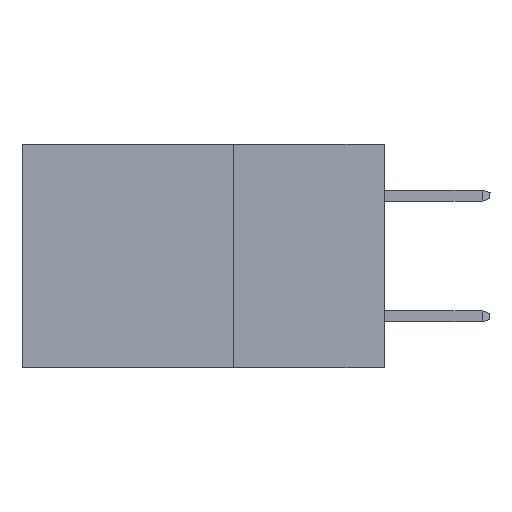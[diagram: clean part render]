
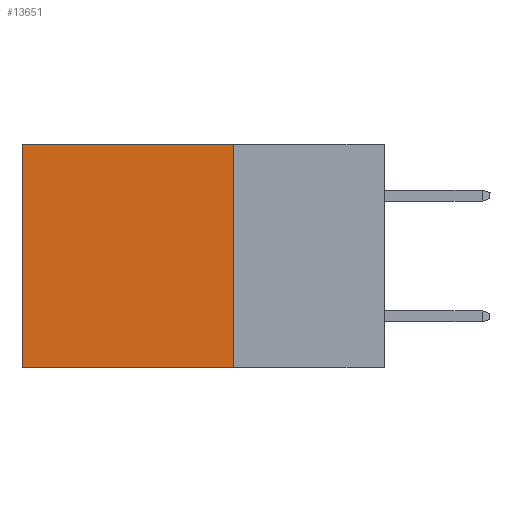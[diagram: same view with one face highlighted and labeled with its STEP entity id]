
A CAD part, left-side view. The second image highlights one B-rep face of the part: STEP entity #13651.
In plain terms, the highlighted planar face has unit normal (-1, 0, 0).
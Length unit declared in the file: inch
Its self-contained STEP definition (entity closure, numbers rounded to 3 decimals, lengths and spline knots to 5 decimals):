
#188 = VERTEX_POINT ( 'NONE', #18555 ) ;
#229 = VERTEX_POINT ( 'NONE', #8361 ) ;
#421 = LINE ( 'NONE', #22026, #21901 ) ;
#2353 = PLANE ( 'NONE',  #11314 ) ;
#4172 = DIRECTION ( 'NONE',  ( 0., 0., -1. ) ) ;
#4690 = CARTESIAN_POINT ( 'NONE',  ( 0.2615, 0.6, 0. ) ) ;
#5053 = CARTESIAN_POINT ( 'NONE',  ( 0.2615, 0.25, 0. ) ) ;
#6602 = ORIENTED_EDGE ( 'NONE', *, *, #17754, .T. ) ;
#6830 = VECTOR ( 'NONE', #22351, 39.37008 ) ;
#7051 = EDGE_CURVE ( 'NONE', #21820, #188, #18152, .T. ) ;
#7388 = DIRECTION ( 'NONE',  ( 0., 0., -1. ) ) ;
#7572 = EDGE_LOOP ( 'NONE', ( #11608, #9899, #9314, #6602 ) ) ;
#7646 = CARTESIAN_POINT ( 'NONE',  ( 0.2615, 0.25, -0.37 ) ) ;
#7740 = FACE_OUTER_BOUND ( 'NONE', #7572, .T. ) ;
#7822 = VERTEX_POINT ( 'NONE', #4690 ) ;
#8204 = CARTESIAN_POINT ( 'NONE',  ( 0.2615, 0.6, -0.37 ) ) ;
#8361 = CARTESIAN_POINT ( 'NONE',  ( 0.2615, 0.25, 0. ) ) ;
#9314 = ORIENTED_EDGE ( 'NONE', *, *, #18350, .F. ) ;
#9574 = EDGE_CURVE ( 'NONE', #7822, #188, #20826, .T. ) ;
#9899 = ORIENTED_EDGE ( 'NONE', *, *, #7051, .F. ) ;
#10002 = DIRECTION ( 'NONE',  ( 0., 0., -1. ) ) ;
#11314 = AXIS2_PLACEMENT_3D ( 'NONE', #7646, #14546, #4172 ) ;
#11608 = ORIENTED_EDGE ( 'NONE', *, *, #9574, .T. ) ;
#13651 = ADVANCED_FACE ( 'NONE', ( #7740 ), #2353, .F. ) ;
#14089 = CARTESIAN_POINT ( 'NONE',  ( 0.2615, 0.25, -0.37 ) ) ;
#14168 = DIRECTION ( 'NONE',  ( 0., 1., 0. ) ) ;
#14546 = DIRECTION ( 'NONE',  ( 1., 0., 0. ) ) ;
#15696 = VECTOR ( 'NONE', #7388, 39.37008 ) ;
#17754 = EDGE_CURVE ( 'NONE', #229, #7822, #20575, .T. ) ;
#18152 = LINE ( 'NONE', #14089, #22204 ) ;
#18350 = EDGE_CURVE ( 'NONE', #229, #21820, #421, .T. ) ;
#18555 = CARTESIAN_POINT ( 'NONE',  ( 0.2615, 0.6, -0.37 ) ) ;
#19709 = CARTESIAN_POINT ( 'NONE',  ( 0.2615, 0.25, -0.37 ) ) ;
#20575 = LINE ( 'NONE', #5053, #6830 ) ;
#20826 = LINE ( 'NONE', #8204, #15696 ) ;
#21820 = VERTEX_POINT ( 'NONE', #19709 ) ;
#21901 = VECTOR ( 'NONE', #10002, 39.37008 ) ;
#22026 = CARTESIAN_POINT ( 'NONE',  ( 0.2615, 0.25, -0.37 ) ) ;
#22204 = VECTOR ( 'NONE', #14168, 39.37008 ) ;
#22351 = DIRECTION ( 'NONE',  ( 0., 1., 0. ) ) ;
